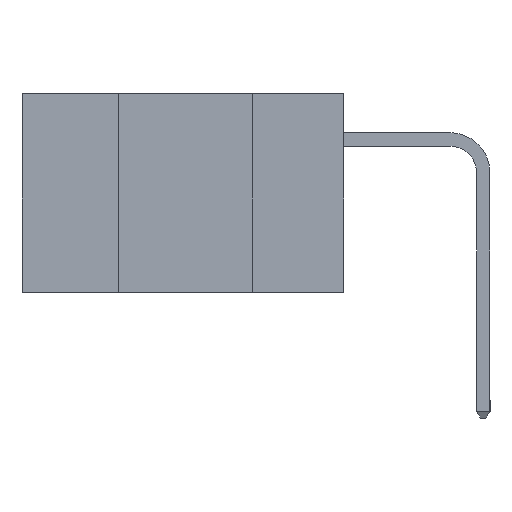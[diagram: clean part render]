
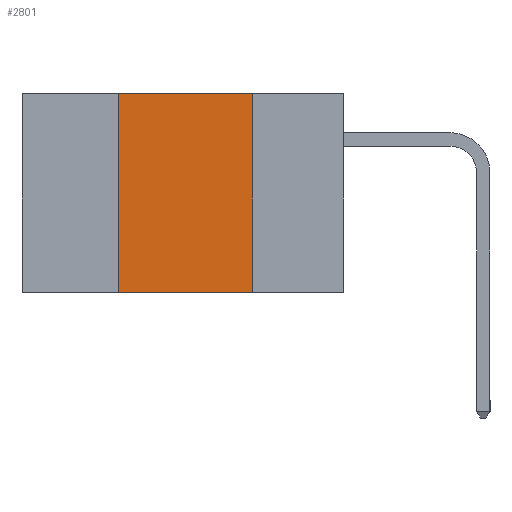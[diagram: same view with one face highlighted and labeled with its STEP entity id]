
A CAD part, left-side view. The second image highlights one B-rep face of the part: STEP entity #2801.
In plain terms, the highlighted planar face has unit normal (-1, 0, 0).
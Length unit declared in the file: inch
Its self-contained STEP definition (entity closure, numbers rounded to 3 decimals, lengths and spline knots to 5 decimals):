
#48 = ORIENTED_EDGE ( 'NONE', *, *, #1803, .F. ) ;
#58 = CARTESIAN_POINT ( 'NONE',  ( 0., 0.17, -0.37 ) ) ;
#337 = ORIENTED_EDGE ( 'NONE', *, *, #14303, .F. ) ;
#529 = LINE ( 'NONE', #11432, #10423 ) ;
#828 = EDGE_CURVE ( 'NONE', #8818, #12718, #5597, .T. ) ;
#1319 = VERTEX_POINT ( 'NONE', #10245 ) ;
#1803 = EDGE_CURVE ( 'NONE', #1319, #3999, #3681, .T. ) ;
#2736 = EDGE_CURVE ( 'NONE', #8818, #1319, #529, .T. ) ;
#2801 = ADVANCED_FACE ( 'NONE', ( #9637 ), #8016, .F. ) ;
#2806 = VECTOR ( 'NONE', #12830, 39.37008 ) ;
#3681 = LINE ( 'NONE', #11952, #2806 ) ;
#3999 = VERTEX_POINT ( 'NONE', #5829 ) ;
#4546 = ORIENTED_EDGE ( 'NONE', *, *, #2736, .F. ) ;
#4964 = ORIENTED_EDGE ( 'NONE', *, *, #828, .T. ) ;
#5328 = AXIS2_PLACEMENT_3D ( 'NONE', #13512, #15429, #15497 ) ;
#5597 = LINE ( 'NONE', #11539, #15644 ) ;
#5829 = CARTESIAN_POINT ( 'NONE',  ( 0., 0.17, 0. ) ) ;
#7810 = CARTESIAN_POINT ( 'NONE',  ( 0., 0.17, -0.37 ) ) ;
#8016 = PLANE ( 'NONE',  #5328 ) ;
#8251 = VECTOR ( 'NONE', #10428, 39.37008 ) ;
#8818 = VERTEX_POINT ( 'NONE', #9593 ) ;
#9593 = CARTESIAN_POINT ( 'NONE',  ( 0., 0.42, -0.37 ) ) ;
#9637 = FACE_OUTER_BOUND ( 'NONE', #10784, .T. ) ;
#10245 = CARTESIAN_POINT ( 'NONE',  ( 0., 0.42, 0. ) ) ;
#10423 = VECTOR ( 'NONE', #16647, 39.37008 ) ;
#10428 = DIRECTION ( 'NONE',  ( 0., 0., -1. ) ) ;
#10784 = EDGE_LOOP ( 'NONE', ( #337, #48, #4546, #4964 ) ) ;
#11432 = CARTESIAN_POINT ( 'NONE',  ( 0., 0.42, -0.37 ) ) ;
#11539 = CARTESIAN_POINT ( 'NONE',  ( 0., 0.6, -0.37 ) ) ;
#11634 = LINE ( 'NONE', #7810, #8251 ) ;
#11952 = CARTESIAN_POINT ( 'NONE',  ( 0., 0.6, 0. ) ) ;
#12718 = VERTEX_POINT ( 'NONE', #58 ) ;
#12830 = DIRECTION ( 'NONE',  ( 0., -1., 0. ) ) ;
#13512 = CARTESIAN_POINT ( 'NONE',  ( 0., 0.6, 0. ) ) ;
#14303 = EDGE_CURVE ( 'NONE', #3999, #12718, #11634, .T. ) ;
#15272 = DIRECTION ( 'NONE',  ( 0., -1., 0. ) ) ;
#15429 = DIRECTION ( 'NONE',  ( 1., 0., 0. ) ) ;
#15497 = DIRECTION ( 'NONE',  ( 0., 0., -1. ) ) ;
#15644 = VECTOR ( 'NONE', #15272, 39.37008 ) ;
#16647 = DIRECTION ( 'NONE',  ( 0., 0., 1. ) ) ;
